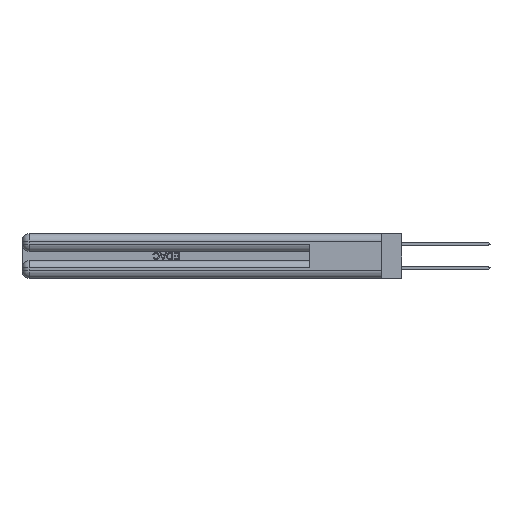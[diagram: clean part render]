
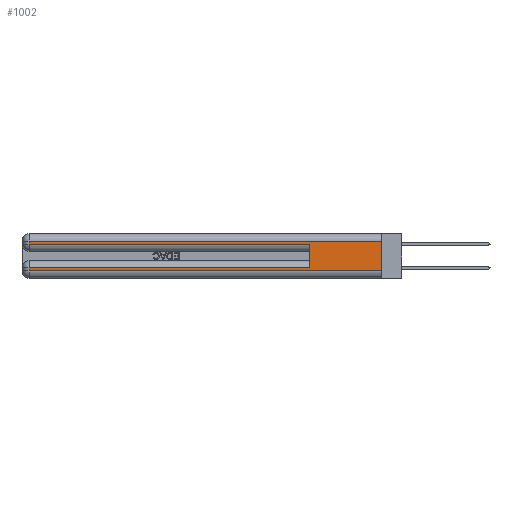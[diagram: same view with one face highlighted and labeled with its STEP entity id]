
A CAD part, left-side view. The second image highlights one B-rep face of the part: STEP entity #1002.
In plain terms, the highlighted planar face has unit normal (-1, 0, 0).
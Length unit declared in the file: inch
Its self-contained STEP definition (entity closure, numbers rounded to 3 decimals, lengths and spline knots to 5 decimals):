
#729 = VERTEX_POINT ( 'NONE', #50864 ) ;
#1002 = ADVANCED_FACE ( 'NONE', ( #7371 ), #7045, .F. ) ;
#1201 = CARTESIAN_POINT ( 'NONE',  ( 0., 0.6, 0.085 ) ) ;
#1422 = EDGE_LOOP ( 'NONE', ( #21921, #29797, #28846, #41843, #35385, #33694, #53071, #45764 ) ) ;
#1761 = LINE ( 'NONE', #44453, #32443 ) ;
#2193 = AXIS2_PLACEMENT_3D ( 'NONE', #15555, #7233, #36277 ) ;
#3147 = CARTESIAN_POINT ( 'NONE',  ( 0., 2.94, 0.31 ) ) ;
#3217 = CARTESIAN_POINT ( 'NONE',  ( 0., 2.94, 0.085 ) ) ;
#4703 = EDGE_CURVE ( 'NONE', #729, #23832, #4916, .T. ) ;
#4916 = LINE ( 'NONE', #6456, #23241 ) ;
#5984 = CARTESIAN_POINT ( 'NONE',  ( 0., 0., 0.085 ) ) ;
#6456 = CARTESIAN_POINT ( 'NONE',  ( 0., 0., 0.37 ) ) ;
#7045 = PLANE ( 'NONE',  #2193 ) ;
#7233 = DIRECTION ( 'NONE',  ( 1., 0., 0. ) ) ;
#7371 = FACE_OUTER_BOUND ( 'NONE', #1422, .T. ) ;
#7966 = DIRECTION ( 'NONE',  ( 0., 0., -1. ) ) ;
#8620 = LINE ( 'NONE', #38346, #39096 ) ;
#9082 = EDGE_CURVE ( 'NONE', #729, #32999, #25562, .T. ) ;
#10606 = EDGE_CURVE ( 'NONE', #32999, #14548, #1761, .T. ) ;
#11282 = EDGE_CURVE ( 'NONE', #12238, #23832, #43958, .T. ) ;
#12238 = VERTEX_POINT ( 'NONE', #35820 ) ;
#13230 = VECTOR ( 'NONE', #31091, 39.37008 ) ;
#14516 = VECTOR ( 'NONE', #30549, 39.37008 ) ;
#14548 = VERTEX_POINT ( 'NONE', #26138 ) ;
#15555 = CARTESIAN_POINT ( 'NONE',  ( 0., 0., 0.37 ) ) ;
#16462 = CARTESIAN_POINT ( 'NONE',  ( 0., 2.94, 0.37 ) ) ;
#17463 = VERTEX_POINT ( 'NONE', #1201 ) ;
#17600 = VERTEX_POINT ( 'NONE', #43894 ) ;
#17819 = DIRECTION ( 'NONE',  ( 0., 0., 1. ) ) ;
#17992 = DIRECTION ( 'NONE',  ( 0., -1., 0. ) ) ;
#19115 = VECTOR ( 'NONE', #17992, 39.37008 ) ;
#19926 = CARTESIAN_POINT ( 'NONE',  ( 0., 0., 0.06 ) ) ;
#21921 = ORIENTED_EDGE ( 'NONE', *, *, #4703, .F. ) ;
#23241 = VECTOR ( 'NONE', #31375, 39.37008 ) ;
#23295 = EDGE_CURVE ( 'NONE', #14548, #17600, #50661, .T. ) ;
#23832 = VERTEX_POINT ( 'NONE', #33591 ) ;
#24385 = VECTOR ( 'NONE', #7966, 39.37008 ) ;
#25562 = LINE ( 'NONE', #42805, #14516 ) ;
#26138 = CARTESIAN_POINT ( 'NONE',  ( 0., 2.94, 0.285 ) ) ;
#27814 = EDGE_CURVE ( 'NONE', #31080, #12238, #47526, .T. ) ;
#28587 = EDGE_CURVE ( 'NONE', #17463, #17600, #8620, .T. ) ;
#28846 = ORIENTED_EDGE ( 'NONE', *, *, #10606, .T. ) ;
#29797 = ORIENTED_EDGE ( 'NONE', *, *, #9082, .T. ) ;
#30240 = CARTESIAN_POINT ( 'NONE',  ( 0., 0., 0.285 ) ) ;
#30549 = DIRECTION ( 'NONE',  ( 0., 1., 0. ) ) ;
#31080 = VERTEX_POINT ( 'NONE', #3217 ) ;
#31091 = DIRECTION ( 'NONE',  ( 0., 1., 0. ) ) ;
#31375 = DIRECTION ( 'NONE',  ( 0., 0., -1. ) ) ;
#32443 = VECTOR ( 'NONE', #36336, 39.37008 ) ;
#32999 = VERTEX_POINT ( 'NONE', #3147 ) ;
#33591 = CARTESIAN_POINT ( 'NONE',  ( 0., 0., 0.06 ) ) ;
#33694 = ORIENTED_EDGE ( 'NONE', *, *, #51108, .T. ) ;
#35173 = LINE ( 'NONE', #5984, #13230 ) ;
#35385 = ORIENTED_EDGE ( 'NONE', *, *, #28587, .F. ) ;
#35820 = CARTESIAN_POINT ( 'NONE',  ( 0., 2.94, 0.06 ) ) ;
#36277 = DIRECTION ( 'NONE',  ( 0., 0., -1. ) ) ;
#36336 = DIRECTION ( 'NONE',  ( 0., 0., -1. ) ) ;
#38346 = CARTESIAN_POINT ( 'NONE',  ( 0., 0.6, 0.145 ) ) ;
#39096 = VECTOR ( 'NONE', #17819, 39.37008 ) ;
#40440 = DIRECTION ( 'NONE',  ( 0., -1., 0. ) ) ;
#41843 = ORIENTED_EDGE ( 'NONE', *, *, #23295, .T. ) ;
#42690 = VECTOR ( 'NONE', #40440, 39.37008 ) ;
#42805 = CARTESIAN_POINT ( 'NONE',  ( 0., 0., 0.31 ) ) ;
#43894 = CARTESIAN_POINT ( 'NONE',  ( 0., 0.6, 0.285 ) ) ;
#43958 = LINE ( 'NONE', #19926, #42690 ) ;
#44453 = CARTESIAN_POINT ( 'NONE',  ( 0., 2.94, 0.37 ) ) ;
#45764 = ORIENTED_EDGE ( 'NONE', *, *, #11282, .T. ) ;
#47526 = LINE ( 'NONE', #16462, #24385 ) ;
#50661 = LINE ( 'NONE', #30240, #19115 ) ;
#50864 = CARTESIAN_POINT ( 'NONE',  ( 0., 0., 0.31 ) ) ;
#51108 = EDGE_CURVE ( 'NONE', #17463, #31080, #35173, .T. ) ;
#53071 = ORIENTED_EDGE ( 'NONE', *, *, #27814, .T. ) ;
